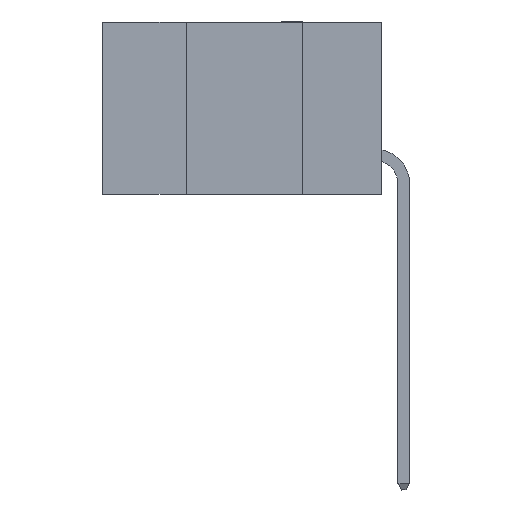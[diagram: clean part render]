
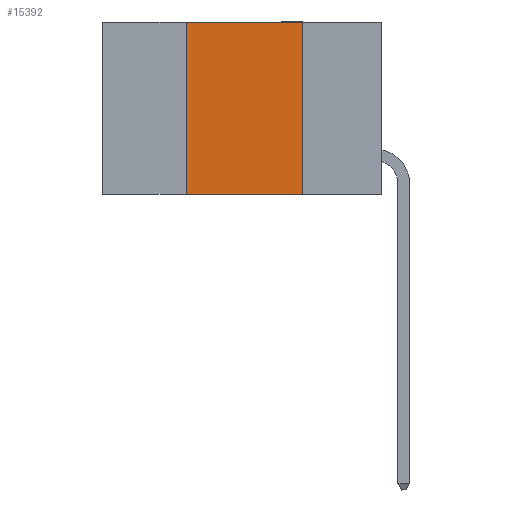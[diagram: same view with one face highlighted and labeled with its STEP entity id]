
A CAD part, left-side view. The second image highlights one B-rep face of the part: STEP entity #15392.
In plain terms, the highlighted planar face has unit normal (-1, 0, 0).
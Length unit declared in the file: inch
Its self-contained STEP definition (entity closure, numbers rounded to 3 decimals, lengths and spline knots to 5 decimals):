
#591 = VECTOR ( 'NONE', #15009, 39.37008 ) ;
#1237 = CARTESIAN_POINT ( 'NONE',  ( 0., 0.6, 0. ) ) ;
#1486 = CARTESIAN_POINT ( 'NONE',  ( 0., 0.17, 0. ) ) ;
#2092 = CARTESIAN_POINT ( 'NONE',  ( 0., 0.6, -0.37 ) ) ;
#2110 = PLANE ( 'NONE',  #4824 ) ;
#3335 = DIRECTION ( 'NONE',  ( 0., 0., 1. ) ) ;
#3378 = CARTESIAN_POINT ( 'NONE',  ( 0., 0.42, 0. ) ) ;
#3484 = CARTESIAN_POINT ( 'NONE',  ( 0., 0.42, 0. ) ) ;
#3790 = ORIENTED_EDGE ( 'NONE', *, *, #7453, .F. ) ;
#4233 = VERTEX_POINT ( 'NONE', #8502 ) ;
#4410 = VECTOR ( 'NONE', #12034, 39.37008 ) ;
#4824 = AXIS2_PLACEMENT_3D ( 'NONE', #10542, #10591, #5728 ) ;
#5493 = DIRECTION ( 'NONE',  ( 0., -1., 0. ) ) ;
#5728 = DIRECTION ( 'NONE',  ( 0., 0., -1. ) ) ;
#5939 = LINE ( 'NONE', #12621, #591 ) ;
#6565 = VERTEX_POINT ( 'NONE', #1486 ) ;
#6943 = VERTEX_POINT ( 'NONE', #14587 ) ;
#7297 = ORIENTED_EDGE ( 'NONE', *, *, #8986, .F. ) ;
#7453 = EDGE_CURVE ( 'NONE', #6943, #13557, #13380, .T. ) ;
#7586 = EDGE_LOOP ( 'NONE', ( #7297, #13480, #3790, #12872 ) ) ;
#8202 = LINE ( 'NONE', #2092, #12372 ) ;
#8502 = CARTESIAN_POINT ( 'NONE',  ( 0., 0.17, -0.37 ) ) ;
#8986 = EDGE_CURVE ( 'NONE', #6565, #4233, #5939, .T. ) ;
#9290 = FACE_OUTER_BOUND ( 'NONE', #7586, .T. ) ;
#10542 = CARTESIAN_POINT ( 'NONE',  ( 0., 0.6, 0. ) ) ;
#10591 = DIRECTION ( 'NONE',  ( 1., 0., 0. ) ) ;
#12034 = DIRECTION ( 'NONE',  ( 0., -1., 0. ) ) ;
#12372 = VECTOR ( 'NONE', #5493, 39.37008 ) ;
#12621 = CARTESIAN_POINT ( 'NONE',  ( 0., 0.17, 0. ) ) ;
#12872 = ORIENTED_EDGE ( 'NONE', *, *, #13517, .T. ) ;
#13202 = VECTOR ( 'NONE', #3335, 39.37008 ) ;
#13380 = LINE ( 'NONE', #3484, #13202 ) ;
#13407 = EDGE_CURVE ( 'NONE', #13557, #6565, #15241, .T. ) ;
#13480 = ORIENTED_EDGE ( 'NONE', *, *, #13407, .F. ) ;
#13517 = EDGE_CURVE ( 'NONE', #6943, #4233, #8202, .T. ) ;
#13557 = VERTEX_POINT ( 'NONE', #3378 ) ;
#14587 = CARTESIAN_POINT ( 'NONE',  ( 0., 0.42, -0.37 ) ) ;
#15009 = DIRECTION ( 'NONE',  ( 0., 0., -1. ) ) ;
#15241 = LINE ( 'NONE', #1237, #4410 ) ;
#15392 = ADVANCED_FACE ( 'NONE', ( #9290 ), #2110, .F. ) ;
